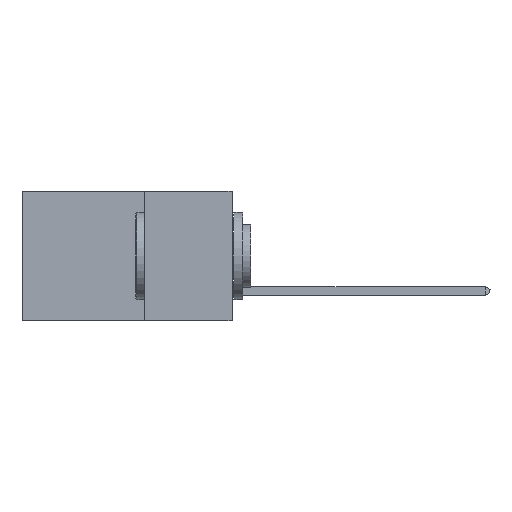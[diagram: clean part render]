
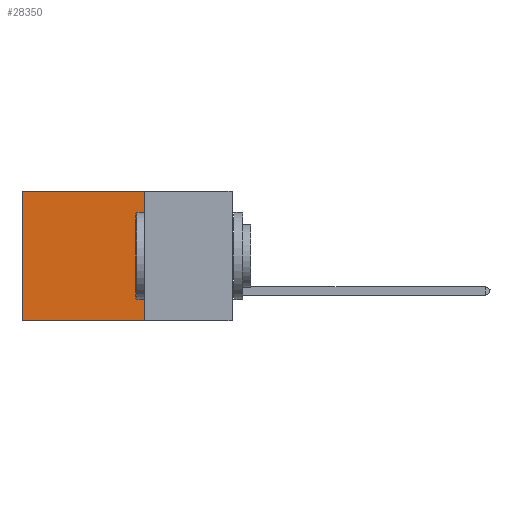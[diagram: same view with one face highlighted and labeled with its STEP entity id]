
A CAD part, left-side view. The second image highlights one B-rep face of the part: STEP entity #28350.
In plain terms, the highlighted planar face has unit normal (-1, 0, 0).
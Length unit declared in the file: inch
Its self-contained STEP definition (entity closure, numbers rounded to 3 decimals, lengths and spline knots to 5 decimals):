
#1039 = ORIENTED_EDGE ( 'NONE', *, *, #18433, .T. ) ;
#1374 = DIRECTION ( 'NONE',  ( 0., 1., 0. ) ) ;
#1624 = CARTESIAN_POINT ( 'NONE',  ( 0.2875, 0.25, 0. ) ) ;
#3425 = VERTEX_POINT ( 'NONE', #6161 ) ;
#3549 = VECTOR ( 'NONE', #30173, 39.37008 ) ;
#6161 = CARTESIAN_POINT ( 'NONE',  ( 0.2875, 0.25, -0.37 ) ) ;
#6467 = LINE ( 'NONE', #14409, #33541 ) ;
#6519 = DIRECTION ( 'NONE',  ( 0., 0., -1. ) ) ;
#6588 = VERTEX_POINT ( 'NONE', #21834 ) ;
#8321 = DIRECTION ( 'NONE',  ( 0., 1., 0. ) ) ;
#8569 = CARTESIAN_POINT ( 'NONE',  ( 0.2875, 0.25, 0. ) ) ;
#10278 = VECTOR ( 'NONE', #1374, 39.37008 ) ;
#11887 = FACE_OUTER_BOUND ( 'NONE', #28714, .T. ) ;
#12298 = VERTEX_POINT ( 'NONE', #1624 ) ;
#12463 = CARTESIAN_POINT ( 'NONE',  ( 0.2875, 0.25, 0. ) ) ;
#12684 = EDGE_CURVE ( 'NONE', #3425, #15392, #6467, .T. ) ;
#14210 = EDGE_CURVE ( 'NONE', #12298, #3425, #22308, .T. ) ;
#14409 = CARTESIAN_POINT ( 'NONE',  ( 0.2875, 0.25, -0.37 ) ) ;
#14903 = DIRECTION ( 'NONE',  ( 0., 0., -1. ) ) ;
#15392 = VERTEX_POINT ( 'NONE', #30978 ) ;
#15711 = AXIS2_PLACEMENT_3D ( 'NONE', #12463, #25634, #14903 ) ;
#17688 = ORIENTED_EDGE ( 'NONE', *, *, #12684, .F. ) ;
#17966 = LINE ( 'NONE', #24571, #3549 ) ;
#18433 = EDGE_CURVE ( 'NONE', #6588, #15392, #17966, .T. ) ;
#19345 = CARTESIAN_POINT ( 'NONE',  ( 0.2875, 0.25, 0. ) ) ;
#19548 = ORIENTED_EDGE ( 'NONE', *, *, #14210, .F. ) ;
#20303 = VECTOR ( 'NONE', #6519, 39.37008 ) ;
#21834 = CARTESIAN_POINT ( 'NONE',  ( 0.2875, 0.6, 0. ) ) ;
#22308 = LINE ( 'NONE', #19345, #20303 ) ;
#24571 = CARTESIAN_POINT ( 'NONE',  ( 0.2875, 0.6, 0. ) ) ;
#25634 = DIRECTION ( 'NONE',  ( 1., 0., 0. ) ) ;
#26420 = ORIENTED_EDGE ( 'NONE', *, *, #32490, .T. ) ;
#26657 = LINE ( 'NONE', #8569, #10278 ) ;
#28350 = ADVANCED_FACE ( 'NONE', ( #11887 ), #30655, .F. ) ;
#28714 = EDGE_LOOP ( 'NONE', ( #1039, #17688, #19548, #26420 ) ) ;
#30173 = DIRECTION ( 'NONE',  ( 0., 0., -1. ) ) ;
#30655 = PLANE ( 'NONE',  #15711 ) ;
#30978 = CARTESIAN_POINT ( 'NONE',  ( 0.2875, 0.6, -0.37 ) ) ;
#32490 = EDGE_CURVE ( 'NONE', #12298, #6588, #26657, .T. ) ;
#33541 = VECTOR ( 'NONE', #8321, 39.37008 ) ;
